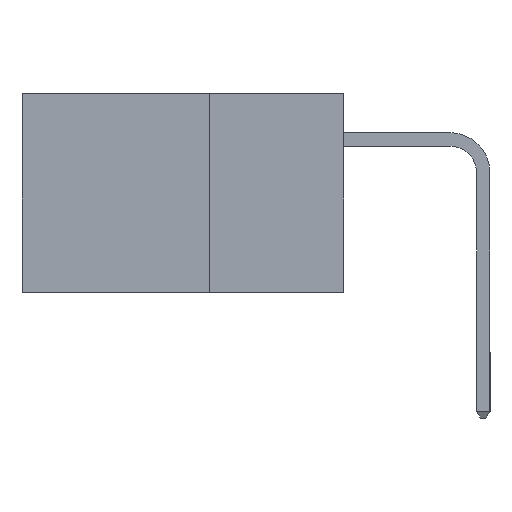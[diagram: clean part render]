
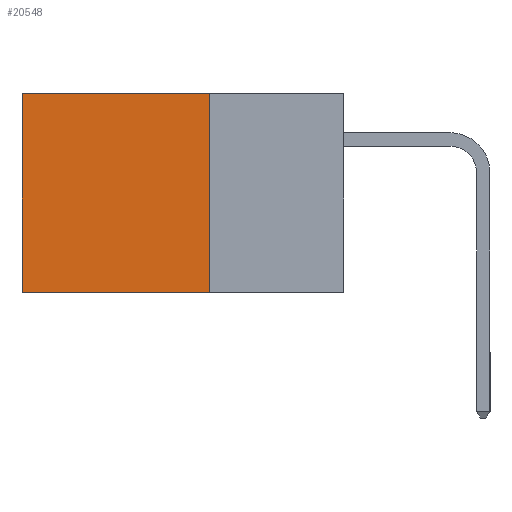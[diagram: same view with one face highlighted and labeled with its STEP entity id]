
A CAD part, left-side view. The second image highlights one B-rep face of the part: STEP entity #20548.
In plain terms, the highlighted planar face has unit normal (-1, 0, 0).
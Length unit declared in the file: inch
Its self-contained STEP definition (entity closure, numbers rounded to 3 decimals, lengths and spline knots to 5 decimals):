
#2374 = ORIENTED_EDGE ( 'NONE', *, *, #3008, .F. ) ;
#2997 = VECTOR ( 'NONE', #13452, 39.37008 ) ;
#3008 = EDGE_CURVE ( 'NONE', #16361, #6934, #18686, .T. ) ;
#4731 = DIRECTION ( 'NONE',  ( 1., 0., 0. ) ) ;
#5947 = CARTESIAN_POINT ( 'NONE',  ( 0.2615, 0.25, -0.37 ) ) ;
#6173 = ORIENTED_EDGE ( 'NONE', *, *, #8613, .T. ) ;
#6636 = DIRECTION ( 'NONE',  ( 0., 0., -1. ) ) ;
#6676 = EDGE_CURVE ( 'NONE', #19989, #11037, #6920, .T. ) ;
#6920 = LINE ( 'NONE', #21500, #11274 ) ;
#6934 = VERTEX_POINT ( 'NONE', #12480 ) ;
#7929 = AXIS2_PLACEMENT_3D ( 'NONE', #10335, #4731, #6636 ) ;
#8497 = ORIENTED_EDGE ( 'NONE', *, *, #6676, .T. ) ;
#8613 = EDGE_CURVE ( 'NONE', #11037, #6934, #17604, .T. ) ;
#8743 = CARTESIAN_POINT ( 'NONE',  ( 0.2615, 0.6, -0.37 ) ) ;
#9042 = VECTOR ( 'NONE', #18942, 39.37008 ) ;
#9169 = DIRECTION ( 'NONE',  ( 0., 1., 0. ) ) ;
#9776 = FACE_OUTER_BOUND ( 'NONE', #15011, .T. ) ;
#9979 = DIRECTION ( 'NONE',  ( 0., 1., 0. ) ) ;
#10335 = CARTESIAN_POINT ( 'NONE',  ( 0.2615, 0.25, -0.37 ) ) ;
#11037 = VERTEX_POINT ( 'NONE', #23002 ) ;
#11274 = VECTOR ( 'NONE', #9979, 39.37008 ) ;
#12480 = CARTESIAN_POINT ( 'NONE',  ( 0.2615, 0.6, -0.37 ) ) ;
#13452 = DIRECTION ( 'NONE',  ( 0., 0., -1. ) ) ;
#14959 = CARTESIAN_POINT ( 'NONE',  ( 0.2615, 0.25, 0. ) ) ;
#15011 = EDGE_LOOP ( 'NONE', ( #6173, #2374, #15753, #8497 ) ) ;
#15231 = CARTESIAN_POINT ( 'NONE',  ( 0.2615, 0.25, -0.37 ) ) ;
#15753 = ORIENTED_EDGE ( 'NONE', *, *, #22220, .F. ) ;
#16361 = VERTEX_POINT ( 'NONE', #21709 ) ;
#17185 = LINE ( 'NONE', #5947, #2997 ) ;
#17351 = VECTOR ( 'NONE', #9169, 39.37008 ) ;
#17604 = LINE ( 'NONE', #8743, #9042 ) ;
#18686 = LINE ( 'NONE', #15231, #17351 ) ;
#18942 = DIRECTION ( 'NONE',  ( 0., 0., -1. ) ) ;
#19989 = VERTEX_POINT ( 'NONE', #14959 ) ;
#20413 = PLANE ( 'NONE',  #7929 ) ;
#20548 = ADVANCED_FACE ( 'NONE', ( #9776 ), #20413, .F. ) ;
#21500 = CARTESIAN_POINT ( 'NONE',  ( 0.2615, 0.25, 0. ) ) ;
#21709 = CARTESIAN_POINT ( 'NONE',  ( 0.2615, 0.25, -0.37 ) ) ;
#22220 = EDGE_CURVE ( 'NONE', #19989, #16361, #17185, .T. ) ;
#23002 = CARTESIAN_POINT ( 'NONE',  ( 0.2615, 0.6, 0. ) ) ;
